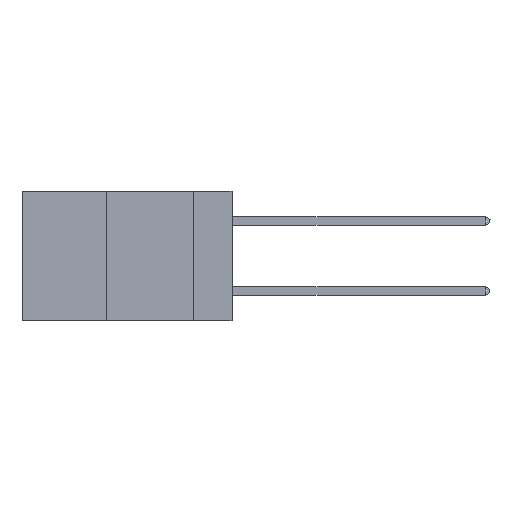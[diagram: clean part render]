
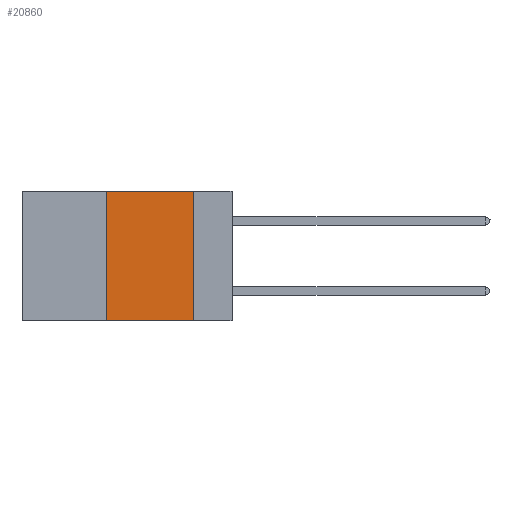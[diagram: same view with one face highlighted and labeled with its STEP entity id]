
A CAD part, left-side view. The second image highlights one B-rep face of the part: STEP entity #20860.
In plain terms, the highlighted planar face has unit normal (-1, 0, 0).
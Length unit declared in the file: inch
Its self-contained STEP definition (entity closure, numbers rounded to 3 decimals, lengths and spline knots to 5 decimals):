
#328 = CARTESIAN_POINT ( 'NONE',  ( 0., 0.11, 0. ) ) ;
#888 = DIRECTION ( 'NONE',  ( 0., 0., 1. ) ) ;
#2284 = EDGE_CURVE ( 'NONE', #15295, #19144, #14667, .T. ) ;
#3239 = ORIENTED_EDGE ( 'NONE', *, *, #18127, .F. ) ;
#3925 = DIRECTION ( 'NONE',  ( 0., -1., 0. ) ) ;
#5959 = DIRECTION ( 'NONE',  ( 1., 0., 0. ) ) ;
#6872 = AXIS2_PLACEMENT_3D ( 'NONE', #14137, #5959, #17410 ) ;
#7176 = ORIENTED_EDGE ( 'NONE', *, *, #15108, .F. ) ;
#7303 = VECTOR ( 'NONE', #12135, 39.37008 ) ;
#7945 = CARTESIAN_POINT ( 'NONE',  ( 0., 0.11, -0.37 ) ) ;
#8797 = EDGE_CURVE ( 'NONE', #9594, #13734, #17113, .T. ) ;
#9594 = VERTEX_POINT ( 'NONE', #13887 ) ;
#10481 = FACE_OUTER_BOUND ( 'NONE', #13538, .T. ) ;
#11817 = CARTESIAN_POINT ( 'NONE',  ( 0., 0.6, 0. ) ) ;
#12135 = DIRECTION ( 'NONE',  ( 0., 0., -1. ) ) ;
#12642 = ORIENTED_EDGE ( 'NONE', *, *, #2284, .T. ) ;
#12874 = VECTOR ( 'NONE', #13417, 39.37008 ) ;
#13417 = DIRECTION ( 'NONE',  ( 0., -1., 0. ) ) ;
#13538 = EDGE_LOOP ( 'NONE', ( #7176, #20131, #3239, #12642 ) ) ;
#13734 = VERTEX_POINT ( 'NONE', #20097 ) ;
#13851 = CARTESIAN_POINT ( 'NONE',  ( 0., 0.6, -0.37 ) ) ;
#13887 = CARTESIAN_POINT ( 'NONE',  ( 0., 0.36, 0. ) ) ;
#14137 = CARTESIAN_POINT ( 'NONE',  ( 0., 0.6, 0. ) ) ;
#14667 = LINE ( 'NONE', #13851, #18428 ) ;
#15108 = EDGE_CURVE ( 'NONE', #13734, #19144, #15470, .T. ) ;
#15295 = VERTEX_POINT ( 'NONE', #20556 ) ;
#15302 = VECTOR ( 'NONE', #888, 39.37008 ) ;
#15470 = LINE ( 'NONE', #328, #7303 ) ;
#15762 = PLANE ( 'NONE',  #6872 ) ;
#17113 = LINE ( 'NONE', #11817, #12874 ) ;
#17410 = DIRECTION ( 'NONE',  ( 0., 0., -1. ) ) ;
#17459 = CARTESIAN_POINT ( 'NONE',  ( 0., 0.36, 0. ) ) ;
#18127 = EDGE_CURVE ( 'NONE', #15295, #9594, #20078, .T. ) ;
#18428 = VECTOR ( 'NONE', #3925, 39.37008 ) ;
#19144 = VERTEX_POINT ( 'NONE', #7945 ) ;
#20078 = LINE ( 'NONE', #17459, #15302 ) ;
#20097 = CARTESIAN_POINT ( 'NONE',  ( 0., 0.11, 0. ) ) ;
#20131 = ORIENTED_EDGE ( 'NONE', *, *, #8797, .F. ) ;
#20556 = CARTESIAN_POINT ( 'NONE',  ( 0., 0.36, -0.37 ) ) ;
#20860 = ADVANCED_FACE ( 'NONE', ( #10481 ), #15762, .F. ) ;
